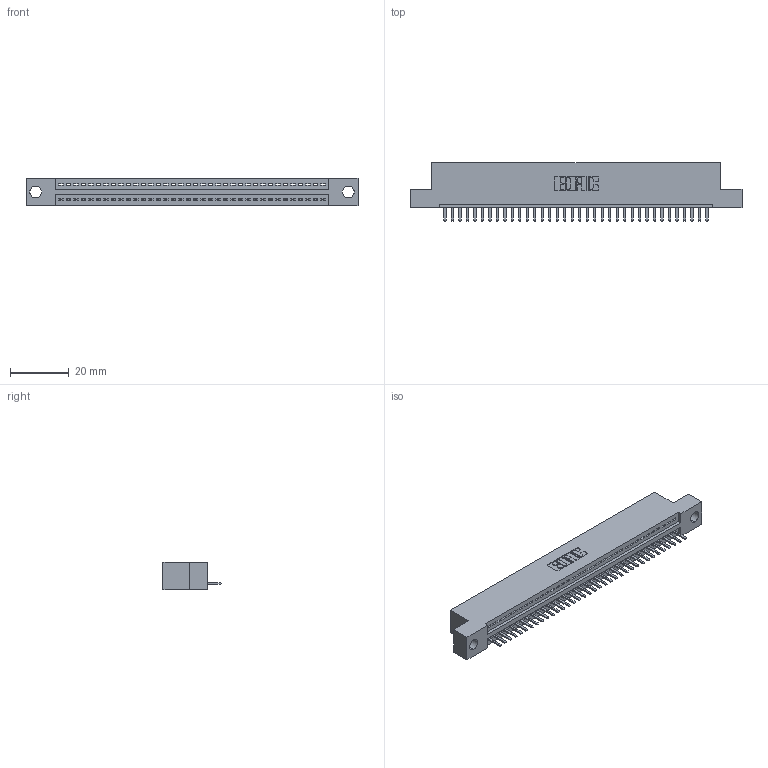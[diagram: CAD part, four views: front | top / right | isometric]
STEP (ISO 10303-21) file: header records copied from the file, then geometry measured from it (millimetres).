
FILE_DESCRIPTION (( 'STEP AP203' ), '1' );
FILE_NAME ('395-036-520-104.STEP', '2021-05-31T14:53:08', ( '' ), ( '' ), 'SwSTEP 2.0', 'SolidWorks 2020', '' );
FILE_SCHEMA (( 'CONFIG_CONTROL_DESIGN' ));
Length unit declared in the file: inch
Products named in the file (3): 395-036-520-104; 345-292-001_345-293-120; 345 Part_Flush Mounting Lugs - 0.156 Dia-TI
Assembly tree (37 placements, depth 2):
  395-036-520-104
    345 Part_Flush Mounting Lugs - 0.156 Dia-TI
    345-292-001_345-293-120  x36
Bounding box: 112.65 x 19.68 x 9.4 mm (x, y, z)
Volume: 10440.9 mm3; surface area: 13297.1 mm2
Topology: 37 solids, 37 shells, 2372 faces, 7001 edges, 4570 vertices
Faces by surface type: plane 1606, cylinder 766
Entity records: 28435 total; most frequent: CARTESIAN_POINT 4946, ORIENTED_EDGE 4902, DIRECTION 4315, EDGE_CURVE 2451, LINE 2171, VECTOR 2171, VERTEX_POINT 1630, AXIS2_PLACEMENT_3D 1072
